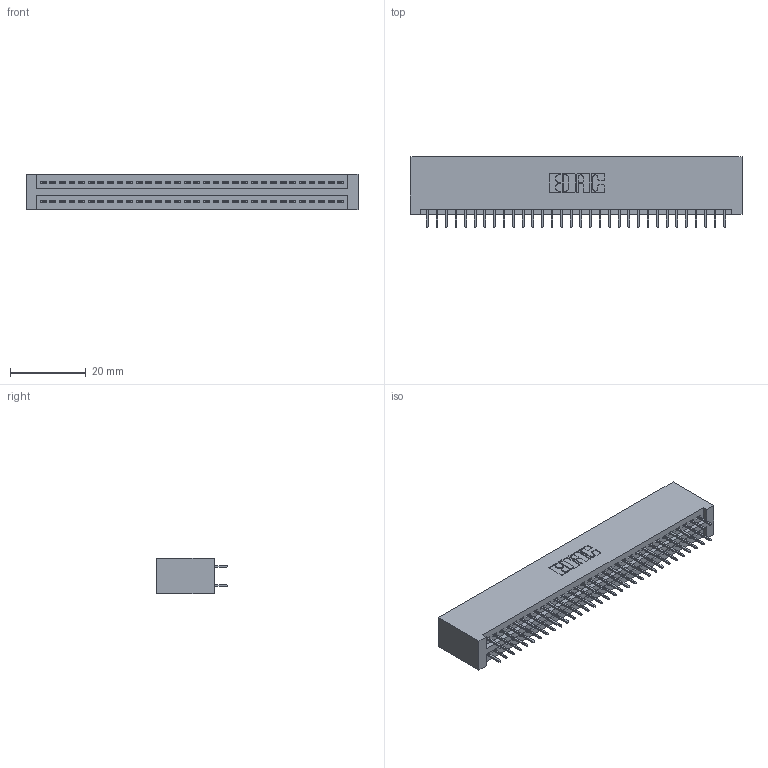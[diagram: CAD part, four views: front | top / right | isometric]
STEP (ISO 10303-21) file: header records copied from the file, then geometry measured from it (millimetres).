
FILE_DESCRIPTION (( 'STEP AP203' ), '1' );
FILE_NAME ('845-064-525-201.STEP', '2020-09-23T17:42:07', ( '' ), ( '' ), 'SwSTEP 2.0', 'SolidWorks 2020', '' );
FILE_SCHEMA (( 'CONFIG_CONTROL_DESIGN' ));
Length unit declared in the file: inch
Products named in the file (3): 845 Part_No Mounting Lugs; 845-064-525-201; 345-292-001_345-293-125
Assembly tree (65 placements, depth 2):
  845-064-525-201
    845 Part_No Mounting Lugs
    345-292-001_345-293-125  x64
Bounding box: 87.88 x 18.72 x 9.4 mm (x, y, z)
Volume: 8954.9 mm3; surface area: 13029 mm2
Topology: 65 solids, 65 shells, 3574 faces, 10109 edges, 6482 vertices
Faces by surface type: plane 2572, cylinder 1002
Entity records: 26251 total; most frequent: CARTESIAN_POINT 4408, ORIENTED_EDGE 4342, DIRECTION 3895, EDGE_CURVE 2171, LINE 1923, VECTOR 1923, VERTEX_POINT 1442, AXIS2_PLACEMENT_3D 986
